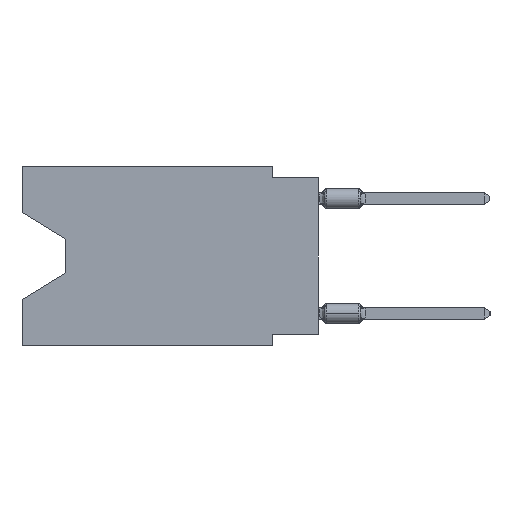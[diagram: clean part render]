
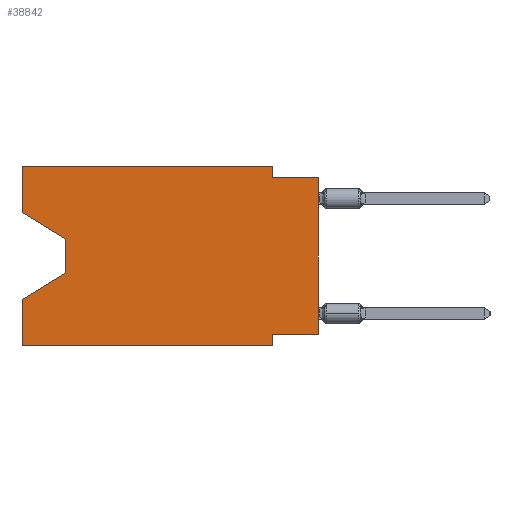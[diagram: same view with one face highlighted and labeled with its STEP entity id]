
A CAD part, left-side view. The second image highlights one B-rep face of the part: STEP entity #38842.
In plain terms, the highlighted planar face has unit normal (-1, 0, 0).
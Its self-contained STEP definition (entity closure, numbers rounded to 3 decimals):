
#72 = EDGE_CURVE ( 'NONE', #2345, #43308, #37165, .T. ) ;
#340 = CARTESIAN_POINT ( 'NONE',  ( 0., 16.383, 0. ) ) ;
#646 = VERTEX_POINT ( 'NONE', #45734 ) ;
#1130 = LINE ( 'NONE', #15929, #19639 ) ;
#2345 = VERTEX_POINT ( 'NONE', #17260 ) ;
#3048 = LINE ( 'NONE', #28561, #19637 ) ;
#4920 = LINE ( 'NONE', #340, #10642 ) ;
#6160 = CARTESIAN_POINT ( 'NONE',  ( 0., 16.383, -7.36 ) ) ;
#6957 = CARTESIAN_POINT ( 'NONE',  ( 0., 13.97, -5.893 ) ) ;
#7151 = DIRECTION ( 'NONE',  ( 0., -1., 0. ) ) ;
#7169 = DIRECTION ( 'NONE',  ( 0., 0., -1. ) ) ;
#7332 = CARTESIAN_POINT ( 'NONE',  ( 0., 0., -9.271 ) ) ;
#7888 = DIRECTION ( 'NONE',  ( 0., 0., -1. ) ) ;
#8241 = ORIENTED_EDGE ( 'NONE', *, *, #26574, .T. ) ;
#9186 = EDGE_CURVE ( 'NONE', #646, #43799, #4920, .T. ) ;
#9587 = ORIENTED_EDGE ( 'NONE', *, *, #32015, .T. ) ;
#10642 = VECTOR ( 'NONE', #19040, 1000. ) ;
#11164 = VERTEX_POINT ( 'NONE', #14558 ) ;
#11644 = ORIENTED_EDGE ( 'NONE', *, *, #33874, .F. ) ;
#11822 = CARTESIAN_POINT ( 'NONE',  ( 0., 0., -9.271 ) ) ;
#11858 = AXIS2_PLACEMENT_3D ( 'NONE', #33073, #21182, #13626 ) ;
#12298 = EDGE_CURVE ( 'NONE', #2345, #27203, #33339, .T. ) ;
#13626 = DIRECTION ( 'NONE',  ( 0., 0., -1. ) ) ;
#13791 = LINE ( 'NONE', #28623, #17943 ) ;
#14204 = LINE ( 'NONE', #29496, #36138 ) ;
#14262 = ORIENTED_EDGE ( 'NONE', *, *, #38115, .F. ) ;
#14558 = CARTESIAN_POINT ( 'NONE',  ( 0., 13.97, -4.013 ) ) ;
#15929 = CARTESIAN_POINT ( 'NONE',  ( 0., 2.54, -9.906 ) ) ;
#16605 = EDGE_CURVE ( 'NONE', #646, #11164, #31048, .T. ) ;
#17151 = EDGE_CURVE ( 'NONE', #29962, #27203, #1130, .T. ) ;
#17260 = CARTESIAN_POINT ( 'NONE',  ( 0., 16.383, -9.906 ) ) ;
#17310 = ORIENTED_EDGE ( 'NONE', *, *, #16605, .T. ) ;
#17943 = VECTOR ( 'NONE', #24985, 1000. ) ;
#19040 = DIRECTION ( 'NONE',  ( 0., 0., 1. ) ) ;
#19419 = VECTOR ( 'NONE', #29938, 1000. ) ;
#19637 = VECTOR ( 'NONE', #47265, 1000. ) ;
#19639 = VECTOR ( 'NONE', #41907, 1000. ) ;
#20378 = DIRECTION ( 'NONE',  ( 0., -0.855, -0.519 ) ) ;
#20381 = VECTOR ( 'NONE', #24715, 1000. ) ;
#20808 = VERTEX_POINT ( 'NONE', #24615 ) ;
#21182 = DIRECTION ( 'NONE',  ( 1., 0., 0. ) ) ;
#21626 = EDGE_CURVE ( 'NONE', #43799, #42685, #3048, .T. ) ;
#22277 = LINE ( 'NONE', #30024, #33475 ) ;
#24615 = CARTESIAN_POINT ( 'NONE',  ( 0., 2.54, -0.635 ) ) ;
#24715 = DIRECTION ( 'NONE',  ( 0., 0.855, -0.519 ) ) ;
#24985 = DIRECTION ( 'NONE',  ( 0., 0., 1. ) ) ;
#25406 = ORIENTED_EDGE ( 'NONE', *, *, #17151, .F. ) ;
#25640 = CARTESIAN_POINT ( 'NONE',  ( 0., 2.54, 0. ) ) ;
#26029 = VECTOR ( 'NONE', #7169, 1000. ) ;
#26246 = VECTOR ( 'NONE', #33505, 1000. ) ;
#26574 = EDGE_CURVE ( 'NONE', #11164, #30300, #22277, .T. ) ;
#26862 = CARTESIAN_POINT ( 'NONE',  ( 0., 13.97, -5.893 ) ) ;
#27203 = VERTEX_POINT ( 'NONE', #46565 ) ;
#28561 = CARTESIAN_POINT ( 'NONE',  ( 0., 16.383, 0. ) ) ;
#28623 = CARTESIAN_POINT ( 'NONE',  ( 0., 0., 0. ) ) ;
#29393 = VERTEX_POINT ( 'NONE', #7332 ) ;
#29496 = CARTESIAN_POINT ( 'NONE',  ( 0., 0., -0.635 ) ) ;
#29938 = DIRECTION ( 'NONE',  ( 0., -1., 0. ) ) ;
#29962 = VERTEX_POINT ( 'NONE', #34200 ) ;
#30024 = CARTESIAN_POINT ( 'NONE',  ( 0., 13.97, -4.013 ) ) ;
#30300 = VERTEX_POINT ( 'NONE', #26862 ) ;
#31048 = LINE ( 'NONE', #38087, #35961 ) ;
#31306 = EDGE_CURVE ( 'NONE', #20808, #40892, #14204, .T. ) ;
#32015 = EDGE_CURVE ( 'NONE', #29393, #40892, #13791, .T. ) ;
#32253 = CARTESIAN_POINT ( 'NONE',  ( 0., 0., -0.635 ) ) ;
#32367 = CARTESIAN_POINT ( 'NONE',  ( 0., 16.383, 0. ) ) ;
#32586 = PLANE ( 'NONE',  #11858 ) ;
#33073 = CARTESIAN_POINT ( 'NONE',  ( 0., 16.383, 0. ) ) ;
#33339 = LINE ( 'NONE', #43550, #19419 ) ;
#33475 = VECTOR ( 'NONE', #7888, 1000. ) ;
#33505 = DIRECTION ( 'NONE',  ( 0., 0., 1. ) ) ;
#33803 = ORIENTED_EDGE ( 'NONE', *, *, #72, .F. ) ;
#33874 = EDGE_CURVE ( 'NONE', #42685, #20808, #43873, .T. ) ;
#34200 = CARTESIAN_POINT ( 'NONE',  ( 0., 2.54, -9.271 ) ) ;
#34676 = ORIENTED_EDGE ( 'NONE', *, *, #31306, .F. ) ;
#35961 = VECTOR ( 'NONE', #20378, 1000. ) ;
#36138 = VECTOR ( 'NONE', #7151, 1000. ) ;
#36453 = CARTESIAN_POINT ( 'NONE',  ( 0., 2.54, 0. ) ) ;
#37165 = LINE ( 'NONE', #47871, #26246 ) ;
#38087 = CARTESIAN_POINT ( 'NONE',  ( 0., 16.383, -2.546 ) ) ;
#38115 = EDGE_CURVE ( 'NONE', #29393, #29962, #45123, .T. ) ;
#38842 = ADVANCED_FACE ( 'NONE', ( #39617 ), #32586, .F. ) ;
#39617 = FACE_OUTER_BOUND ( 'NONE', #47970, .T. ) ;
#39786 = VECTOR ( 'NONE', #41493, 1000. ) ;
#40890 = EDGE_CURVE ( 'NONE', #30300, #43308, #43171, .T. ) ;
#40892 = VERTEX_POINT ( 'NONE', #32253 ) ;
#41493 = DIRECTION ( 'NONE',  ( 0., 1., 0. ) ) ;
#41907 = DIRECTION ( 'NONE',  ( 0., 0., -1. ) ) ;
#42533 = ORIENTED_EDGE ( 'NONE', *, *, #9186, .F. ) ;
#42685 = VERTEX_POINT ( 'NONE', #36453 ) ;
#43171 = LINE ( 'NONE', #6957, #20381 ) ;
#43308 = VERTEX_POINT ( 'NONE', #6160 ) ;
#43521 = ORIENTED_EDGE ( 'NONE', *, *, #21626, .F. ) ;
#43550 = CARTESIAN_POINT ( 'NONE',  ( 0., 16.383, -9.906 ) ) ;
#43799 = VERTEX_POINT ( 'NONE', #32367 ) ;
#43873 = LINE ( 'NONE', #25640, #26029 ) ;
#44671 = ORIENTED_EDGE ( 'NONE', *, *, #40890, .T. ) ;
#45123 = LINE ( 'NONE', #11822, #39786 ) ;
#45173 = ORIENTED_EDGE ( 'NONE', *, *, #12298, .T. ) ;
#45734 = CARTESIAN_POINT ( 'NONE',  ( 0., 16.383, -2.546 ) ) ;
#46565 = CARTESIAN_POINT ( 'NONE',  ( 0., 2.54, -9.906 ) ) ;
#47265 = DIRECTION ( 'NONE',  ( 0., -1., 0. ) ) ;
#47871 = CARTESIAN_POINT ( 'NONE',  ( 0., 16.383, 0. ) ) ;
#47970 = EDGE_LOOP ( 'NONE', ( #17310, #8241, #44671, #33803, #45173, #25406, #14262, #9587, #34676, #11644, #43521, #42533 ) ) ;
